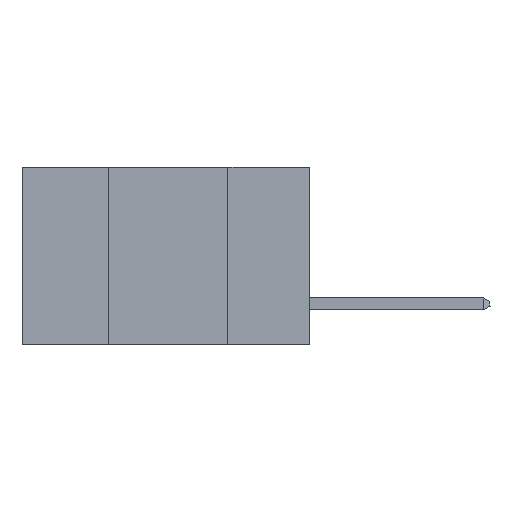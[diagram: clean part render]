
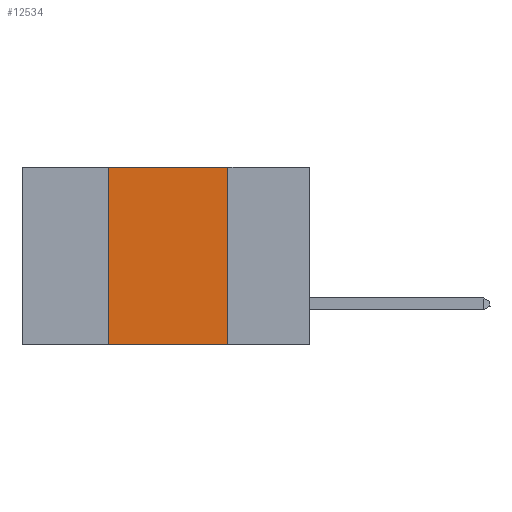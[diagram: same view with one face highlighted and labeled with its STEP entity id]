
A CAD part, left-side view. The second image highlights one B-rep face of the part: STEP entity #12534.
In plain terms, the highlighted planar face has unit normal (-1, 0, 0).
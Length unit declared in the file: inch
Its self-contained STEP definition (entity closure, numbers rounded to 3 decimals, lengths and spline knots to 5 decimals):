
#479 = ORIENTED_EDGE ( 'NONE', *, *, #7405, .F. ) ;
#1471 = CARTESIAN_POINT ( 'NONE',  ( 0., 0.17, 0. ) ) ;
#1547 = CARTESIAN_POINT ( 'NONE',  ( 0., 0.6, 0. ) ) ;
#2326 = CARTESIAN_POINT ( 'NONE',  ( 0., 0.6, 0. ) ) ;
#2404 = CARTESIAN_POINT ( 'NONE',  ( 0., 0.17, -0.37 ) ) ;
#2405 = AXIS2_PLACEMENT_3D ( 'NONE', #2326, #10620, #11925 ) ;
#2407 = FACE_OUTER_BOUND ( 'NONE', #7395, .T. ) ;
#2791 = DIRECTION ( 'NONE',  ( 0., -1., 0. ) ) ;
#4123 = ORIENTED_EDGE ( 'NONE', *, *, #15152, .F. ) ;
#4595 = DIRECTION ( 'NONE',  ( 0., 0., 1. ) ) ;
#5875 = VERTEX_POINT ( 'NONE', #12972 ) ;
#6121 = LINE ( 'NONE', #16852, #6536 ) ;
#6122 = VERTEX_POINT ( 'NONE', #16393 ) ;
#6536 = VECTOR ( 'NONE', #4595, 39.37008 ) ;
#6649 = CARTESIAN_POINT ( 'NONE',  ( 0., 0.17, 0. ) ) ;
#7134 = EDGE_CURVE ( 'NONE', #5875, #6122, #6121, .T. ) ;
#7395 = EDGE_LOOP ( 'NONE', ( #4123, #479, #8361, #13879 ) ) ;
#7405 = EDGE_CURVE ( 'NONE', #6122, #10018, #11630, .T. ) ;
#7822 = LINE ( 'NONE', #6649, #11017 ) ;
#8361 = ORIENTED_EDGE ( 'NONE', *, *, #7134, .F. ) ;
#9218 = PLANE ( 'NONE',  #2405 ) ;
#10018 = VERTEX_POINT ( 'NONE', #1471 ) ;
#10505 = LINE ( 'NONE', #15243, #14291 ) ;
#10620 = DIRECTION ( 'NONE',  ( 1., 0., 0. ) ) ;
#11017 = VECTOR ( 'NONE', #12109, 39.37008 ) ;
#11606 = EDGE_CURVE ( 'NONE', #5875, #17012, #10505, .T. ) ;
#11630 = LINE ( 'NONE', #1547, #14770 ) ;
#11925 = DIRECTION ( 'NONE',  ( 0., 0., -1. ) ) ;
#12109 = DIRECTION ( 'NONE',  ( 0., 0., -1. ) ) ;
#12534 = ADVANCED_FACE ( 'NONE', ( #2407 ), #9218, .F. ) ;
#12972 = CARTESIAN_POINT ( 'NONE',  ( 0., 0.42, -0.37 ) ) ;
#13879 = ORIENTED_EDGE ( 'NONE', *, *, #11606, .T. ) ;
#14291 = VECTOR ( 'NONE', #16617, 39.37008 ) ;
#14770 = VECTOR ( 'NONE', #2791, 39.37008 ) ;
#15152 = EDGE_CURVE ( 'NONE', #10018, #17012, #7822, .T. ) ;
#15243 = CARTESIAN_POINT ( 'NONE',  ( 0., 0.6, -0.37 ) ) ;
#16393 = CARTESIAN_POINT ( 'NONE',  ( 0., 0.42, 0. ) ) ;
#16617 = DIRECTION ( 'NONE',  ( 0., -1., 0. ) ) ;
#16852 = CARTESIAN_POINT ( 'NONE',  ( 0., 0.42, 0. ) ) ;
#17012 = VERTEX_POINT ( 'NONE', #2404 ) ;
